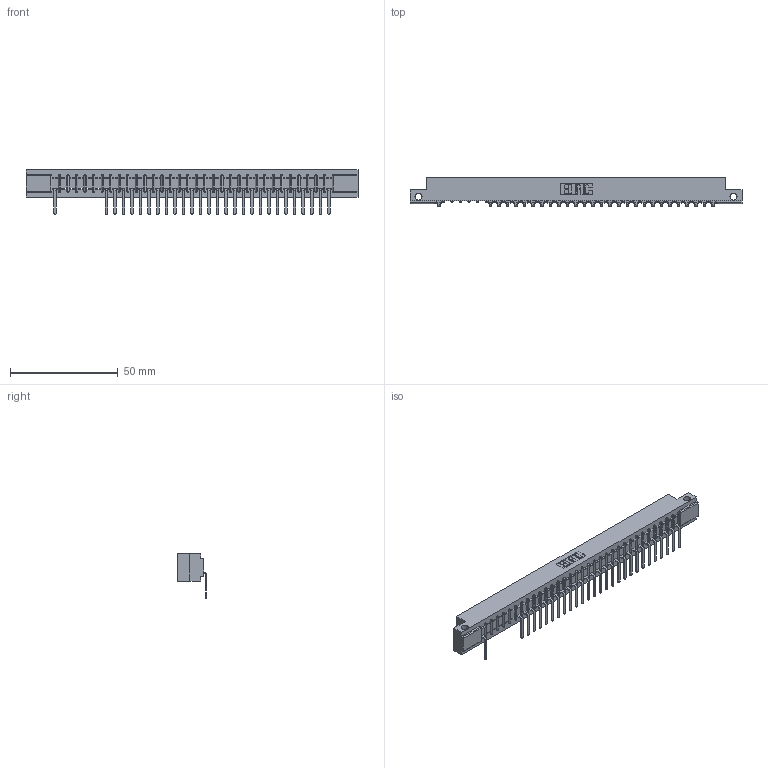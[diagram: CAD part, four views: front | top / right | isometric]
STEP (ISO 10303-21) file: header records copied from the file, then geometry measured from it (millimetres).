
FILE_DESCRIPTION (( 'STEP AP203' ), '1' );
FILE_NAME ('357-033-557-112.STEP', '2018-08-10T01:44:47', ( '' ), ( '' ), 'SwSTEP 2.0', 'SolidWorks 2016', '' );
FILE_SCHEMA (( 'CONFIG_CONTROL_DESIGN' ));
Length unit declared in the file: inch
Products named in the file (3): 357-033-557-112; 307 Part_.128 Dia Side Mounting Holes; 307-290-002_557
Assembly tree (29 placements, depth 2):
  357-033-557-112
    307 Part_.128 Dia Side Mounting Holes
    307-290-002_557  x28
Bounding box: 153.77 x 13.32 x 20.66 mm (x, y, z)
Volume: 16177.2 mm3; surface area: 19696.9 mm2
Topology: 29 solids, 29 shells, 2436 faces, 7475 edges, 4890 vertices
Faces by surface type: plane 1446, cylinder 922, sphere 68
Entity records: 30096 total; most frequent: CARTESIAN_POINT 5099, ORIENTED_EDGE 5094, DIRECTION 4953, EDGE_CURVE 2547, LINE 1945, VECTOR 1945, VERTEX_POINT 1650, AXIS2_PLACEMENT_3D 1504
